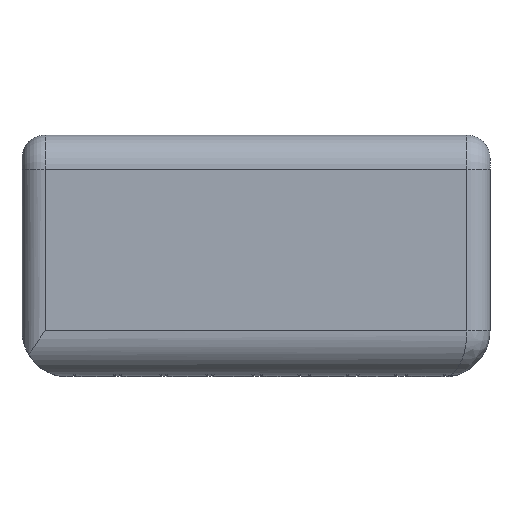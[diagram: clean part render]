
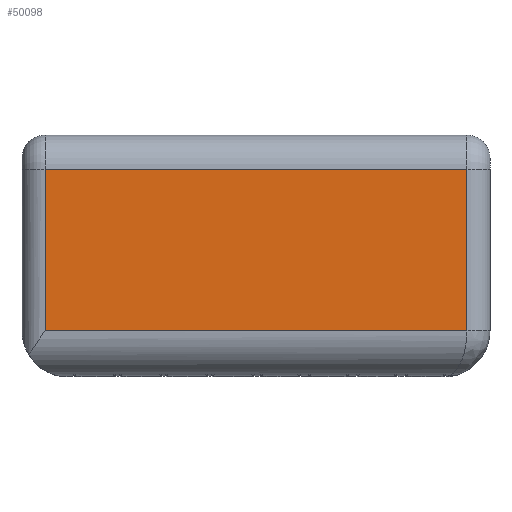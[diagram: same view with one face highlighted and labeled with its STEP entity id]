
A CAD part, left-side view. The second image highlights one B-rep face of the part: STEP entity #50098.
In plain terms, the highlighted planar face has unit normal (-1, 0, 0).
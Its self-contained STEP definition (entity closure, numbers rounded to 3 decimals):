
#4259 = VECTOR ( 'NONE', #28967, 1000. ) ;
#5290 = DIRECTION ( 'NONE',  ( 0., 0., -1. ) ) ;
#5626 = FACE_OUTER_BOUND ( 'NONE', #43358, .T. ) ;
#12118 = AXIS2_PLACEMENT_3D ( 'NONE', #30087, #42537, #5290 ) ;
#12763 = VERTEX_POINT ( 'NONE', #48465 ) ;
#14543 = DIRECTION ( 'NONE',  ( 0., -1., 0. ) ) ;
#19067 = CARTESIAN_POINT ( 'NONE',  ( -25., 5., 16.294 ) ) ;
#28486 = EDGE_CURVE ( 'NONE', #12763, #69501, #71609, .T. ) ;
#28967 = DIRECTION ( 'NONE',  ( 0., 0., 1. ) ) ;
#30087 = CARTESIAN_POINT ( 'NONE',  ( -25., -49.812, 0. ) ) ;
#32339 = ORIENTED_EDGE ( 'NONE', *, *, #34265, .T. ) ;
#32647 = VECTOR ( 'NONE', #66639, 1000. ) ;
#34265 = EDGE_CURVE ( 'NONE', #69501, #50513, #51118, .T. ) ;
#34644 = VECTOR ( 'NONE', #14543, 1000. ) ;
#41338 = CARTESIAN_POINT ( 'NONE',  ( -25., 96.6, -18.706 ) ) ;
#41672 = CARTESIAN_POINT ( 'NONE',  ( -25., 5., 0. ) ) ;
#42537 = DIRECTION ( 'NONE',  ( 1., 0., 0. ) ) ;
#43187 = LINE ( 'NONE', #41672, #4259 ) ;
#43358 = EDGE_LOOP ( 'NONE', ( #32339, #53441, #63280, #50898 ) ) ;
#44839 = EDGE_CURVE ( 'NONE', #70193, #12763, #58680, .T. ) ;
#45342 = CARTESIAN_POINT ( 'NONE',  ( -25., 5., -18.706 ) ) ;
#48465 = CARTESIAN_POINT ( 'NONE',  ( -25., 96.6, 16.294 ) ) ;
#50098 = ADVANCED_FACE ( 'NONE', ( #5626 ), #54787, .F. ) ;
#50513 = VERTEX_POINT ( 'NONE', #45342 ) ;
#50898 = ORIENTED_EDGE ( 'NONE', *, *, #28486, .T. ) ;
#51118 = LINE ( 'NONE', #70555, #34644 ) ;
#53441 = ORIENTED_EDGE ( 'NONE', *, *, #57182, .T. ) ;
#54787 = PLANE ( 'NONE',  #12118 ) ;
#57182 = EDGE_CURVE ( 'NONE', #50513, #70193, #43187, .T. ) ;
#58680 = LINE ( 'NONE', #79756, #73297 ) ;
#63280 = ORIENTED_EDGE ( 'NONE', *, *, #44839, .T. ) ;
#66639 = DIRECTION ( 'NONE',  ( 0., 0., -1. ) ) ;
#69501 = VERTEX_POINT ( 'NONE', #73628 ) ;
#70193 = VERTEX_POINT ( 'NONE', #19067 ) ;
#70555 = CARTESIAN_POINT ( 'NONE',  ( -25., 0., -18.706 ) ) ;
#71609 = LINE ( 'NONE', #41338, #32647 ) ;
#73297 = VECTOR ( 'NONE', #79495, 1000. ) ;
#73628 = CARTESIAN_POINT ( 'NONE',  ( -25., 96.6, -18.706 ) ) ;
#79495 = DIRECTION ( 'NONE',  ( 0., 1., 0. ) ) ;
#79756 = CARTESIAN_POINT ( 'NONE',  ( -25., -49.812, 16.294 ) ) ;
